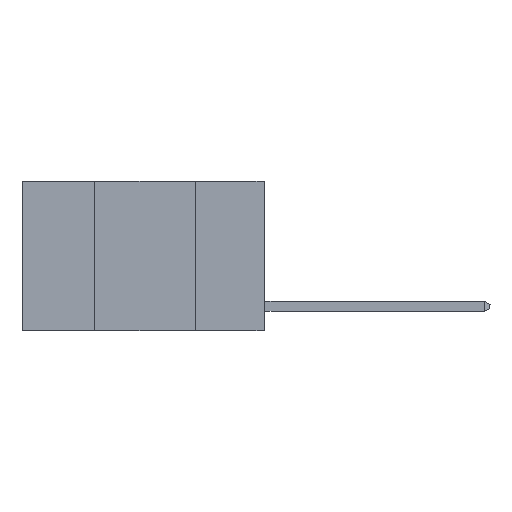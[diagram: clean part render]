
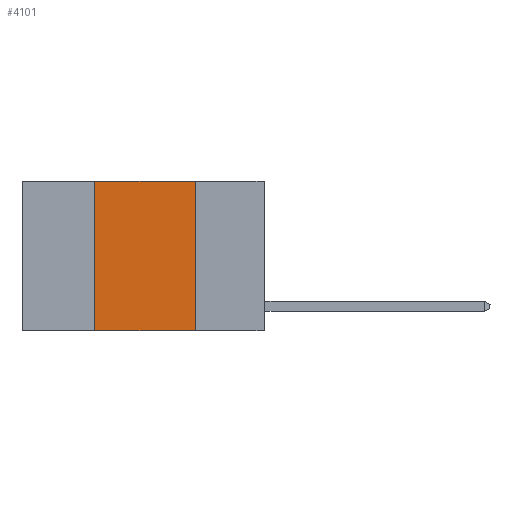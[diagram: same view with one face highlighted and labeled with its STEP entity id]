
A CAD part, left-side view. The second image highlights one B-rep face of the part: STEP entity #4101.
In plain terms, the highlighted planar face has unit normal (-1, 0, 0).
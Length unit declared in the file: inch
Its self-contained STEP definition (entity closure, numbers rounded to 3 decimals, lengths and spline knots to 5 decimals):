
#346 = DIRECTION ( 'NONE',  ( 0., 0., -1. ) ) ;
#417 = EDGE_LOOP ( 'NONE', ( #21029, #21761, #8375, #16985 ) ) ;
#723 = DIRECTION ( 'NONE',  ( 0., 0., -1. ) ) ;
#861 = LINE ( 'NONE', #7362, #25406 ) ;
#1354 = LINE ( 'NONE', #17714, #6932 ) ;
#1672 = CARTESIAN_POINT ( 'NONE',  ( 0., 0.42, 0. ) ) ;
#4101 = ADVANCED_FACE ( 'NONE', ( #17358 ), #21701, .F. ) ;
#4984 = LINE ( 'NONE', #1672, #10498 ) ;
#5549 = CARTESIAN_POINT ( 'NONE',  ( 0., 0.42, -0.37 ) ) ;
#6932 = VECTOR ( 'NONE', #20099, 39.37008 ) ;
#7362 = CARTESIAN_POINT ( 'NONE',  ( 0., 0.6, -0.37 ) ) ;
#8057 = VERTEX_POINT ( 'NONE', #28704 ) ;
#8375 = ORIENTED_EDGE ( 'NONE', *, *, #13161, .F. ) ;
#8776 = AXIS2_PLACEMENT_3D ( 'NONE', #28840, #14643, #346 ) ;
#9709 = VECTOR ( 'NONE', #723, 39.37008 ) ;
#10498 = VECTOR ( 'NONE', #20698, 39.37008 ) ;
#13161 = EDGE_CURVE ( 'NONE', #19257, #18712, #4984, .T. ) ;
#14643 = DIRECTION ( 'NONE',  ( 1., 0., 0. ) ) ;
#14768 = EDGE_CURVE ( 'NONE', #8057, #26549, #28697, .T. ) ;
#15010 = CARTESIAN_POINT ( 'NONE',  ( 0., 0.17, 0. ) ) ;
#16969 = EDGE_CURVE ( 'NONE', #19257, #26549, #861, .T. ) ;
#16985 = ORIENTED_EDGE ( 'NONE', *, *, #16969, .T. ) ;
#17358 = FACE_OUTER_BOUND ( 'NONE', #417, .T. ) ;
#17714 = CARTESIAN_POINT ( 'NONE',  ( 0., 0.6, 0. ) ) ;
#18712 = VERTEX_POINT ( 'NONE', #24879 ) ;
#19257 = VERTEX_POINT ( 'NONE', #5549 ) ;
#20099 = DIRECTION ( 'NONE',  ( 0., -1., 0. ) ) ;
#20698 = DIRECTION ( 'NONE',  ( 0., 0., 1. ) ) ;
#21029 = ORIENTED_EDGE ( 'NONE', *, *, #14768, .F. ) ;
#21624 = DIRECTION ( 'NONE',  ( 0., -1., 0. ) ) ;
#21701 = PLANE ( 'NONE',  #8776 ) ;
#21761 = ORIENTED_EDGE ( 'NONE', *, *, #26580, .F. ) ;
#22379 = CARTESIAN_POINT ( 'NONE',  ( 0., 0.17, -0.37 ) ) ;
#24879 = CARTESIAN_POINT ( 'NONE',  ( 0., 0.42, 0. ) ) ;
#25406 = VECTOR ( 'NONE', #21624, 39.37008 ) ;
#26549 = VERTEX_POINT ( 'NONE', #22379 ) ;
#26580 = EDGE_CURVE ( 'NONE', #18712, #8057, #1354, .T. ) ;
#28697 = LINE ( 'NONE', #15010, #9709 ) ;
#28704 = CARTESIAN_POINT ( 'NONE',  ( 0., 0.17, 0. ) ) ;
#28840 = CARTESIAN_POINT ( 'NONE',  ( 0., 0.6, 0. ) ) ;
